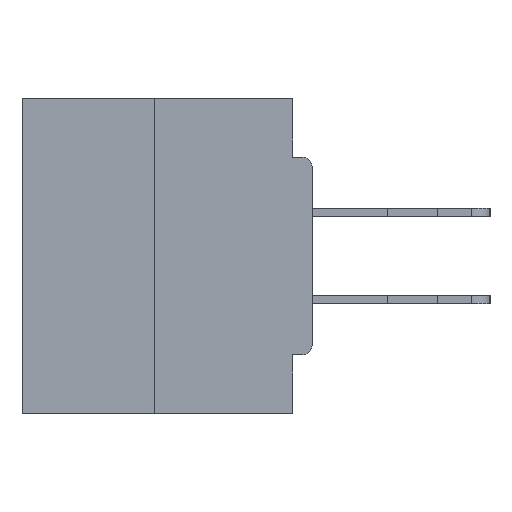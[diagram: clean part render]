
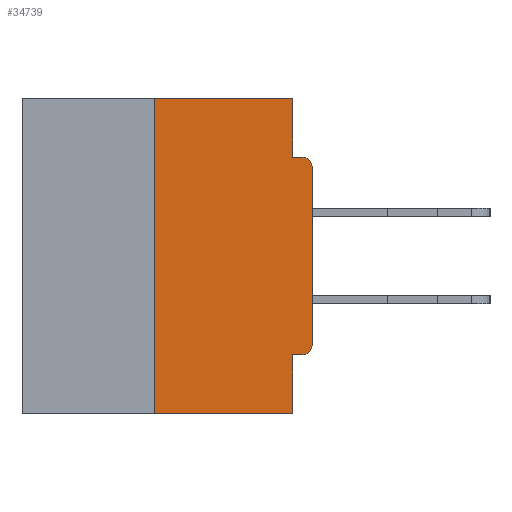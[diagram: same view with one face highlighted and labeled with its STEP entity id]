
A CAD part, left-side view. The second image highlights one B-rep face of the part: STEP entity #34739.
In plain terms, the highlighted planar face has unit normal (-1, 0, 0).
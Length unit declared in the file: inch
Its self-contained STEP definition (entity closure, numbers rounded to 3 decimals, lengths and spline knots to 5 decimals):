
#100 = CARTESIAN_POINT ( 'NONE',  ( 0., 0.46, -0.5 ) ) ;
#763 = CARTESIAN_POINT ( 'NONE',  ( 0., 0.031, 0. ) ) ;
#878 = CARTESIAN_POINT ( 'NONE',  ( 0., 0.015, -0.0935 ) ) ;
#1215 = EDGE_CURVE ( 'NONE', #32997, #5216, #29726, .T. ) ;
#1364 = CARTESIAN_POINT ( 'NONE',  ( 0., 0., -0.0935 ) ) ;
#1689 = VECTOR ( 'NONE', #13280, 39.37008 ) ;
#1863 = VECTOR ( 'NONE', #25139, 39.37008 ) ;
#1890 = LINE ( 'NONE', #1364, #34779 ) ;
#2290 = EDGE_CURVE ( 'NONE', #19962, #15322, #34163, .T. ) ;
#2401 = EDGE_CURVE ( 'NONE', #14320, #14866, #17910, .T. ) ;
#3055 = PLANE ( 'NONE',  #18646 ) ;
#3058 = VECTOR ( 'NONE', #29973, 39.37008 ) ;
#4379 = CARTESIAN_POINT ( 'NONE',  ( 0., 0.031, 0. ) ) ;
#4693 = EDGE_CURVE ( 'NONE', #14866, #19962, #21123, .T. ) ;
#5216 = VERTEX_POINT ( 'NONE', #24549 ) ;
#6494 = FACE_OUTER_BOUND ( 'NONE', #31681, .T. ) ;
#7539 = LINE ( 'NONE', #20000, #1863 ) ;
#7944 = ORIENTED_EDGE ( 'NONE', *, *, #23918, .T. ) ;
#8850 = CARTESIAN_POINT ( 'NONE',  ( 0., 0.015, -0.4065 ) ) ;
#8926 = DIRECTION ( 'NONE',  ( 0., -1., 0. ) ) ;
#9121 = CARTESIAN_POINT ( 'NONE',  ( 0., 0.46, 0. ) ) ;
#9282 = VERTEX_POINT ( 'NONE', #29062 ) ;
#9487 = ORIENTED_EDGE ( 'NONE', *, *, #34453, .T. ) ;
#10358 = EDGE_CURVE ( 'NONE', #15322, #16766, #1890, .T. ) ;
#11583 = DIRECTION ( 'NONE',  ( 1., 0., 0. ) ) ;
#12438 = ORIENTED_EDGE ( 'NONE', *, *, #4693, .F. ) ;
#13094 = CIRCLE ( 'NONE', #17863, 0.015 ) ;
#13280 = DIRECTION ( 'NONE',  ( 0., 0., 1. ) ) ;
#13306 = CARTESIAN_POINT ( 'NONE',  ( 0., 0.25, 0. ) ) ;
#13755 = CARTESIAN_POINT ( 'NONE',  ( 0., 0.031, -0.5 ) ) ;
#14320 = VERTEX_POINT ( 'NONE', #32350 ) ;
#14371 = VERTEX_POINT ( 'NONE', #8850 ) ;
#14409 = ORIENTED_EDGE ( 'NONE', *, *, #10358, .F. ) ;
#14450 = CIRCLE ( 'NONE', #34615, 0.015 ) ;
#14866 = VERTEX_POINT ( 'NONE', #29251 ) ;
#15322 = VERTEX_POINT ( 'NONE', #31591 ) ;
#15355 = EDGE_CURVE ( 'NONE', #14320, #5216, #26275, .T. ) ;
#15518 = EDGE_CURVE ( 'NONE', #26869, #16766, #13094, .T. ) ;
#16766 = VERTEX_POINT ( 'NONE', #878 ) ;
#17223 = ORIENTED_EDGE ( 'NONE', *, *, #15355, .T. ) ;
#17701 = ORIENTED_EDGE ( 'NONE', *, *, #31831, .F. ) ;
#17863 = AXIS2_PLACEMENT_3D ( 'NONE', #19308, #24940, #34384 ) ;
#17910 = LINE ( 'NONE', #13306, #3058 ) ;
#18646 = AXIS2_PLACEMENT_3D ( 'NONE', #19777, #11583, #31290 ) ;
#19308 = CARTESIAN_POINT ( 'NONE',  ( 0., 0.015, -0.1085 ) ) ;
#19676 = CARTESIAN_POINT ( 'NONE',  ( 0., 0.031, -0.4065 ) ) ;
#19777 = CARTESIAN_POINT ( 'NONE',  ( 0., 0.46, 0. ) ) ;
#19962 = VERTEX_POINT ( 'NONE', #763 ) ;
#20000 = CARTESIAN_POINT ( 'NONE',  ( 0., 0., -0.4065 ) ) ;
#20670 = VECTOR ( 'NONE', #25980, 39.37008 ) ;
#21062 = ORIENTED_EDGE ( 'NONE', *, *, #1215, .F. ) ;
#21123 = LINE ( 'NONE', #9121, #20670 ) ;
#21189 = ORIENTED_EDGE ( 'NONE', *, *, #2290, .F. ) ;
#21321 = ORIENTED_EDGE ( 'NONE', *, *, #2401, .F. ) ;
#21388 = CARTESIAN_POINT ( 'NONE',  ( 0., 0.015, -0.3915 ) ) ;
#22110 = DIRECTION ( 'NONE',  ( 0., 0., -1. ) ) ;
#22711 = LINE ( 'NONE', #29825, #1689 ) ;
#23238 = VECTOR ( 'NONE', #8926, 39.37008 ) ;
#23918 = EDGE_CURVE ( 'NONE', #14371, #9282, #14450, .T. ) ;
#24325 = DIRECTION ( 'NONE',  ( 0., 0., -1. ) ) ;
#24439 = CARTESIAN_POINT ( 'NONE',  ( 0., 0., -0.1085 ) ) ;
#24549 = CARTESIAN_POINT ( 'NONE',  ( 0., 0.031, -0.5 ) ) ;
#24940 = DIRECTION ( 'NONE',  ( -1., 0., 0. ) ) ;
#25139 = DIRECTION ( 'NONE',  ( 0., 1., 0. ) ) ;
#25357 = VECTOR ( 'NONE', #26857, 39.37008 ) ;
#25980 = DIRECTION ( 'NONE',  ( 0., -1., 0. ) ) ;
#26275 = LINE ( 'NONE', #100, #23238 ) ;
#26857 = DIRECTION ( 'NONE',  ( 0., 0., -1. ) ) ;
#26869 = VERTEX_POINT ( 'NONE', #24439 ) ;
#27872 = ORIENTED_EDGE ( 'NONE', *, *, #15518, .T. ) ;
#29062 = CARTESIAN_POINT ( 'NONE',  ( 0., 0., -0.3915 ) ) ;
#29251 = CARTESIAN_POINT ( 'NONE',  ( 0., 0.25, 0. ) ) ;
#29726 = LINE ( 'NONE', #13755, #35913 ) ;
#29825 = CARTESIAN_POINT ( 'NONE',  ( 0., 0., 0. ) ) ;
#29844 = DIRECTION ( 'NONE',  ( -1., 0., 0. ) ) ;
#29973 = DIRECTION ( 'NONE',  ( 0., 0., 1. ) ) ;
#31290 = DIRECTION ( 'NONE',  ( 0., 0., -1. ) ) ;
#31591 = CARTESIAN_POINT ( 'NONE',  ( 0., 0.031, -0.0935 ) ) ;
#31681 = EDGE_LOOP ( 'NONE', ( #12438, #21321, #17223, #21062, #17701, #7944, #9487, #27872, #14409, #21189 ) ) ;
#31831 = EDGE_CURVE ( 'NONE', #14371, #32997, #7539, .T. ) ;
#32193 = DIRECTION ( 'NONE',  ( 0., -1., 0. ) ) ;
#32350 = CARTESIAN_POINT ( 'NONE',  ( 0., 0.25, -0.5 ) ) ;
#32997 = VERTEX_POINT ( 'NONE', #19676 ) ;
#34163 = LINE ( 'NONE', #4379, #25357 ) ;
#34384 = DIRECTION ( 'NONE',  ( 0., 0., -1. ) ) ;
#34453 = EDGE_CURVE ( 'NONE', #9282, #26869, #22711, .T. ) ;
#34615 = AXIS2_PLACEMENT_3D ( 'NONE', #21388, #29844, #24325 ) ;
#34739 = ADVANCED_FACE ( 'NONE', ( #6494 ), #3055, .F. ) ;
#34779 = VECTOR ( 'NONE', #32193, 39.37008 ) ;
#35913 = VECTOR ( 'NONE', #22110, 39.37008 ) ;
